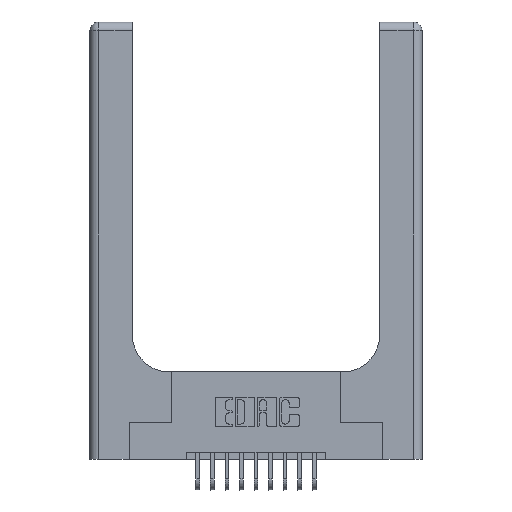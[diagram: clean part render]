
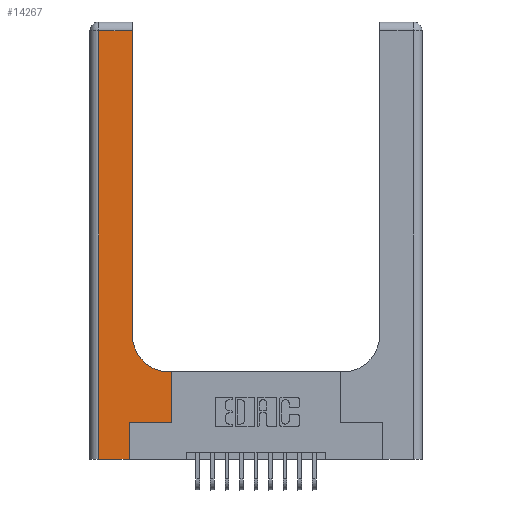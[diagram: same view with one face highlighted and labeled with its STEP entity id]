
A CAD part, top view. The second image highlights one B-rep face of the part: STEP entity #14267.
In plain terms, the highlighted planar face has unit normal (0, 0, 1).
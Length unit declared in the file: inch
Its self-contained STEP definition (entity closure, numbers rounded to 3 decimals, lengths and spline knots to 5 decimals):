
#244 = CARTESIAN_POINT ( 'NONE',  ( 0.06, 2.94, 0.37 ) ) ;
#324 = CARTESIAN_POINT ( 'NONE',  ( 0.5585, 0.6, 0.37 ) ) ;
#373 = VERTEX_POINT ( 'NONE', #16752 ) ;
#402 = CARTESIAN_POINT ( 'NONE',  ( 0.2915, 0.85, 0.37 ) ) ;
#619 = VECTOR ( 'NONE', #9781, 39.37008 ) ;
#1046 = DIRECTION ( 'NONE',  ( -1., 0., 0. ) ) ;
#1299 = LINE ( 'NONE', #17717, #15054 ) ;
#1444 = LINE ( 'NONE', #10342, #12390 ) ;
#1532 = AXIS2_PLACEMENT_3D ( 'NONE', #16251, #3768, #13550 ) ;
#1630 = ORIENTED_EDGE ( 'NONE', *, *, #15942, .T. ) ;
#1810 = CARTESIAN_POINT ( 'NONE',  ( 0.5415, 0.85, 0.37 ) ) ;
#2228 = CARTESIAN_POINT ( 'NONE',  ( 0.2915, 2.94, 0.37 ) ) ;
#2232 = PLANE ( 'NONE',  #1532 ) ;
#2233 = VERTEX_POINT ( 'NONE', #402 ) ;
#2891 = ORIENTED_EDGE ( 'NONE', *, *, #14119, .T. ) ;
#3226 = ORIENTED_EDGE ( 'NONE', *, *, #13102, .T. ) ;
#3345 = DIRECTION ( 'NONE',  ( 0., -1., 0. ) ) ;
#3374 = DIRECTION ( 'NONE',  ( 1., 0., 0. ) ) ;
#3593 = EDGE_CURVE ( 'NONE', #8132, #18027, #7549, .T. ) ;
#3768 = DIRECTION ( 'NONE',  ( 0., 0., -1. ) ) ;
#3883 = CARTESIAN_POINT ( 'NONE',  ( 0.269, 0.25, 0.37 ) ) ;
#3900 = DIRECTION ( 'NONE',  ( 0., 1., 0. ) ) ;
#4012 = VECTOR ( 'NONE', #16351, 39.37008 ) ;
#4397 = ORIENTED_EDGE ( 'NONE', *, *, #11561, .T. ) ;
#4421 = ORIENTED_EDGE ( 'NONE', *, *, #9339, .T. ) ;
#4485 = ORIENTED_EDGE ( 'NONE', *, *, #14481, .T. ) ;
#4925 = CARTESIAN_POINT ( 'NONE',  ( 0.5585, 0.25, 0.37 ) ) ;
#5014 = VERTEX_POINT ( 'NONE', #14541 ) ;
#6093 = VECTOR ( 'NONE', #14622, 39.37008 ) ;
#6222 = VERTEX_POINT ( 'NONE', #244 ) ;
#6512 = VECTOR ( 'NONE', #1046, 39.37008 ) ;
#6803 = DIRECTION ( 'NONE',  ( 0., 1., 0. ) ) ;
#7215 = ORIENTED_EDGE ( 'NONE', *, *, #3593, .T. ) ;
#7337 = VECTOR ( 'NONE', #16318, 39.37008 ) ;
#7549 = LINE ( 'NONE', #12553, #619 ) ;
#7757 = LINE ( 'NONE', #17672, #7337 ) ;
#7790 = LINE ( 'NONE', #3883, #4012 ) ;
#8132 = VERTEX_POINT ( 'NONE', #324 ) ;
#9099 = VECTOR ( 'NONE', #3900, 39.37008 ) ;
#9339 = EDGE_CURVE ( 'NONE', #2233, #16449, #12803, .T. ) ;
#9781 = DIRECTION ( 'NONE',  ( -1., 0., 0. ) ) ;
#10104 = LINE ( 'NONE', #17925, #6512 ) ;
#10342 = CARTESIAN_POINT ( 'NONE',  ( 0.06, 3., 0.37 ) ) ;
#11235 = FACE_OUTER_BOUND ( 'NONE', #13331, .T. ) ;
#11445 = CIRCLE ( 'NONE', #12048, 0.25 ) ;
#11561 = EDGE_CURVE ( 'NONE', #12120, #14898, #7790, .T. ) ;
#11662 = EDGE_CURVE ( 'NONE', #16449, #6222, #10104, .T. ) ;
#11763 = DIRECTION ( 'NONE',  ( 0., 0., -1. ) ) ;
#12048 = AXIS2_PLACEMENT_3D ( 'NONE', #1810, #11763, #3374 ) ;
#12120 = VERTEX_POINT ( 'NONE', #14876 ) ;
#12390 = VECTOR ( 'NONE', #3345, 39.37008 ) ;
#12553 = CARTESIAN_POINT ( 'NONE',  ( 0.2915, 0.6, 0.37 ) ) ;
#12803 = LINE ( 'NONE', #17723, #9099 ) ;
#13102 = EDGE_CURVE ( 'NONE', #6222, #373, #1444, .T. ) ;
#13331 = EDGE_LOOP ( 'NONE', ( #4421, #14166, #3226, #1630, #14679, #4397, #2891, #7215, #4485 ) ) ;
#13550 = DIRECTION ( 'NONE',  ( -1., 0., 0. ) ) ;
#13884 = LINE ( 'NONE', #4925, #6093 ) ;
#14119 = EDGE_CURVE ( 'NONE', #14898, #8132, #13884, .T. ) ;
#14166 = ORIENTED_EDGE ( 'NONE', *, *, #11662, .T. ) ;
#14181 = CARTESIAN_POINT ( 'NONE',  ( 0.5585, 0.25, 0.37 ) ) ;
#14267 = ADVANCED_FACE ( 'NONE', ( #11235 ), #2232, .F. ) ;
#14481 = EDGE_CURVE ( 'NONE', #18027, #2233, #11445, .T. ) ;
#14541 = CARTESIAN_POINT ( 'NONE',  ( 0.269, 0., 0.37 ) ) ;
#14622 = DIRECTION ( 'NONE',  ( 0., 1., 0. ) ) ;
#14679 = ORIENTED_EDGE ( 'NONE', *, *, #17568, .T. ) ;
#14876 = CARTESIAN_POINT ( 'NONE',  ( 0.269, 0.25, 0.37 ) ) ;
#14898 = VERTEX_POINT ( 'NONE', #14181 ) ;
#15054 = VECTOR ( 'NONE', #6803, 39.37008 ) ;
#15942 = EDGE_CURVE ( 'NONE', #373, #5014, #7757, .T. ) ;
#16251 = CARTESIAN_POINT ( 'NONE',  ( 0., 3., 0.37 ) ) ;
#16318 = DIRECTION ( 'NONE',  ( 1., 0., 0. ) ) ;
#16351 = DIRECTION ( 'NONE',  ( 1., 0., 0. ) ) ;
#16449 = VERTEX_POINT ( 'NONE', #2228 ) ;
#16752 = CARTESIAN_POINT ( 'NONE',  ( 0.06, 0., 0.37 ) ) ;
#17275 = CARTESIAN_POINT ( 'NONE',  ( 0.5415, 0.6, 0.37 ) ) ;
#17568 = EDGE_CURVE ( 'NONE', #5014, #12120, #1299, .T. ) ;
#17672 = CARTESIAN_POINT ( 'NONE',  ( 0., 0., 0.37 ) ) ;
#17717 = CARTESIAN_POINT ( 'NONE',  ( 0.269, 0., 0.37 ) ) ;
#17723 = CARTESIAN_POINT ( 'NONE',  ( 0.2915, 3., 0.37 ) ) ;
#17925 = CARTESIAN_POINT ( 'NONE',  ( 0., 2.94, 0.37 ) ) ;
#18027 = VERTEX_POINT ( 'NONE', #17275 ) ;
